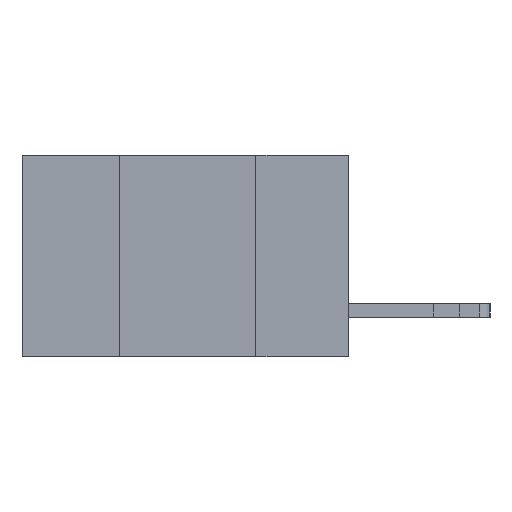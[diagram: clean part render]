
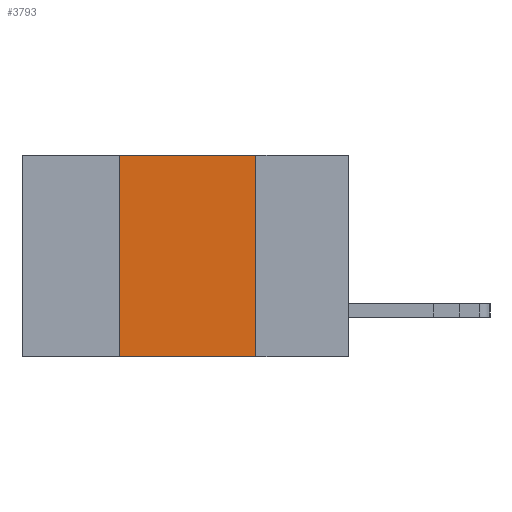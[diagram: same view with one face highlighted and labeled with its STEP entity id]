
A CAD part, left-side view. The second image highlights one B-rep face of the part: STEP entity #3793.
In plain terms, the highlighted planar face has unit normal (-1, 0, 0).
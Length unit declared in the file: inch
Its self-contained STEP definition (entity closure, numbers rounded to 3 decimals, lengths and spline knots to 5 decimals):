
#572 = AXIS2_PLACEMENT_3D ( 'NONE', #7236, #7218, #7196 ) ;
#856 = ORIENTED_EDGE ( 'NONE', *, *, #4761, .T. ) ;
#981 = EDGE_CURVE ( 'NONE', #8211, #9386, #5278, .T. ) ;
#1308 = ORIENTED_EDGE ( 'NONE', *, *, #6582, .F. ) ;
#1622 = EDGE_CURVE ( 'NONE', #9386, #5090, #2659, .T. ) ;
#1818 = CARTESIAN_POINT ( 'NONE',  ( 0., 0.6, 0. ) ) ;
#2659 = LINE ( 'NONE', #3284, #5119 ) ;
#2924 = DIRECTION ( 'NONE',  ( 0., 0., -1. ) ) ;
#3284 = CARTESIAN_POINT ( 'NONE',  ( 0., 0.17, -0.37 ) ) ;
#3793 = ADVANCED_FACE ( 'NONE', ( #8356 ), #7422, .F. ) ;
#4425 = VECTOR ( 'NONE', #4844, 39.37008 ) ;
#4761 = EDGE_CURVE ( 'NONE', #4808, #5090, #5200, .T. ) ;
#4808 = VERTEX_POINT ( 'NONE', #8320 ) ;
#4844 = DIRECTION ( 'NONE',  ( 0., -1., 0. ) ) ;
#4914 = VECTOR ( 'NONE', #8239, 39.37008 ) ;
#5090 = VERTEX_POINT ( 'NONE', #7070 ) ;
#5119 = VECTOR ( 'NONE', #2924, 39.37008 ) ;
#5200 = LINE ( 'NONE', #11823, #4914 ) ;
#5278 = LINE ( 'NONE', #1818, #4425 ) ;
#5768 = VECTOR ( 'NONE', #9192, 39.37008 ) ;
#6269 = ORIENTED_EDGE ( 'NONE', *, *, #1622, .F. ) ;
#6582 = EDGE_CURVE ( 'NONE', #4808, #8211, #8220, .T. ) ;
#7070 = CARTESIAN_POINT ( 'NONE',  ( 0., 0.17, -0.37 ) ) ;
#7196 = DIRECTION ( 'NONE',  ( 0., 0., -1. ) ) ;
#7218 = DIRECTION ( 'NONE',  ( 1., 0., 0. ) ) ;
#7236 = CARTESIAN_POINT ( 'NONE',  ( 0., 0.6, 0. ) ) ;
#7422 = PLANE ( 'NONE',  #572 ) ;
#7896 = CARTESIAN_POINT ( 'NONE',  ( 0., 0.42, 0. ) ) ;
#8211 = VERTEX_POINT ( 'NONE', #7896 ) ;
#8220 = LINE ( 'NONE', #8282, #5768 ) ;
#8239 = DIRECTION ( 'NONE',  ( 0., -1., 0. ) ) ;
#8282 = CARTESIAN_POINT ( 'NONE',  ( 0., 0.42, -0.37 ) ) ;
#8320 = CARTESIAN_POINT ( 'NONE',  ( 0., 0.42, -0.37 ) ) ;
#8356 = FACE_OUTER_BOUND ( 'NONE', #8596, .T. ) ;
#8596 = EDGE_LOOP ( 'NONE', ( #6269, #10001, #1308, #856 ) ) ;
#9192 = DIRECTION ( 'NONE',  ( 0., 0., 1. ) ) ;
#9386 = VERTEX_POINT ( 'NONE', #10379 ) ;
#10001 = ORIENTED_EDGE ( 'NONE', *, *, #981, .F. ) ;
#10379 = CARTESIAN_POINT ( 'NONE',  ( 0., 0.17, 0. ) ) ;
#11823 = CARTESIAN_POINT ( 'NONE',  ( 0., 0.6, -0.37 ) ) ;
